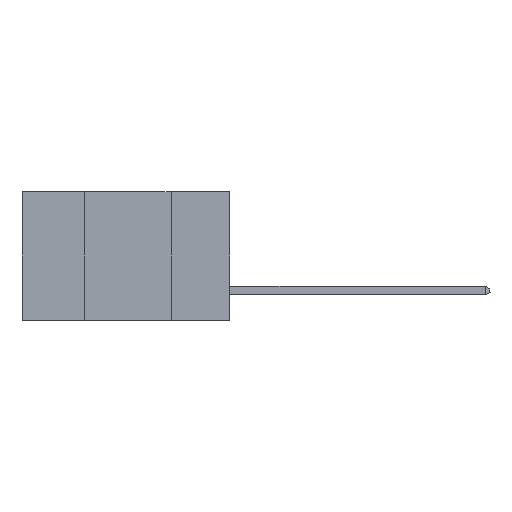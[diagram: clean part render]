
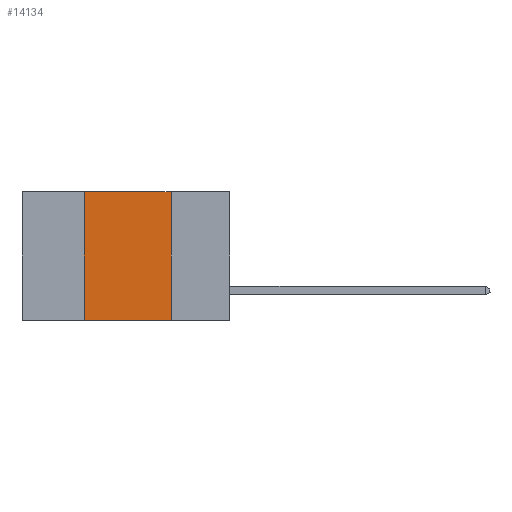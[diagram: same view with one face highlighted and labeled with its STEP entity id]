
A CAD part, left-side view. The second image highlights one B-rep face of the part: STEP entity #14134.
In plain terms, the highlighted planar face has unit normal (-1, 0, 0).
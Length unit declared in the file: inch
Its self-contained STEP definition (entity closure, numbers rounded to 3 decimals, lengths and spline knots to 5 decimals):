
#404 = ORIENTED_EDGE ( 'NONE', *, *, #15050, .F. ) ;
#877 = VECTOR ( 'NONE', #7510, 39.37008 ) ;
#1445 = PLANE ( 'NONE',  #12548 ) ;
#1470 = EDGE_CURVE ( 'NONE', #3828, #5305, #3275, .T. ) ;
#2500 = DIRECTION ( 'NONE',  ( 0., -1., 0. ) ) ;
#2763 = EDGE_CURVE ( 'NONE', #5057, #8301, #10687, .T. ) ;
#3275 = LINE ( 'NONE', #13652, #877 ) ;
#3521 = VECTOR ( 'NONE', #13745, 39.37008 ) ;
#3828 = VERTEX_POINT ( 'NONE', #5385 ) ;
#4058 = EDGE_CURVE ( 'NONE', #5057, #5305, #6656, .T. ) ;
#4372 = CARTESIAN_POINT ( 'NONE',  ( 0., 0.6, -0.37 ) ) ;
#4470 = VECTOR ( 'NONE', #14529, 39.37008 ) ;
#4938 = CARTESIAN_POINT ( 'NONE',  ( 0., 0.17, -0.37 ) ) ;
#5057 = VERTEX_POINT ( 'NONE', #8962 ) ;
#5305 = VERTEX_POINT ( 'NONE', #4938 ) ;
#5385 = CARTESIAN_POINT ( 'NONE',  ( 0., 0.17, 0. ) ) ;
#6128 = ORIENTED_EDGE ( 'NONE', *, *, #1470, .F. ) ;
#6656 = LINE ( 'NONE', #4372, #3521 ) ;
#7510 = DIRECTION ( 'NONE',  ( 0., 0., -1. ) ) ;
#7526 = DIRECTION ( 'NONE',  ( 0., 0., -1. ) ) ;
#8242 = CARTESIAN_POINT ( 'NONE',  ( 0., 0.42, 0. ) ) ;
#8301 = VERTEX_POINT ( 'NONE', #8242 ) ;
#8396 = FACE_OUTER_BOUND ( 'NONE', #14941, .T. ) ;
#8549 = ORIENTED_EDGE ( 'NONE', *, *, #2763, .F. ) ;
#8962 = CARTESIAN_POINT ( 'NONE',  ( 0., 0.42, -0.37 ) ) ;
#9261 = ORIENTED_EDGE ( 'NONE', *, *, #4058, .T. ) ;
#9390 = LINE ( 'NONE', #9516, #11201 ) ;
#9516 = CARTESIAN_POINT ( 'NONE',  ( 0., 0.6, 0. ) ) ;
#9880 = CARTESIAN_POINT ( 'NONE',  ( 0., 0.6, 0. ) ) ;
#10687 = LINE ( 'NONE', #13340, #4470 ) ;
#11201 = VECTOR ( 'NONE', #2500, 39.37008 ) ;
#12548 = AXIS2_PLACEMENT_3D ( 'NONE', #9880, #14541, #7526 ) ;
#13340 = CARTESIAN_POINT ( 'NONE',  ( 0., 0.42, 0. ) ) ;
#13652 = CARTESIAN_POINT ( 'NONE',  ( 0., 0.17, 0. ) ) ;
#13745 = DIRECTION ( 'NONE',  ( 0., -1., 0. ) ) ;
#14134 = ADVANCED_FACE ( 'NONE', ( #8396 ), #1445, .F. ) ;
#14529 = DIRECTION ( 'NONE',  ( 0., 0., 1. ) ) ;
#14541 = DIRECTION ( 'NONE',  ( 1., 0., 0. ) ) ;
#14941 = EDGE_LOOP ( 'NONE', ( #6128, #404, #8549, #9261 ) ) ;
#15050 = EDGE_CURVE ( 'NONE', #8301, #3828, #9390, .T. ) ;
